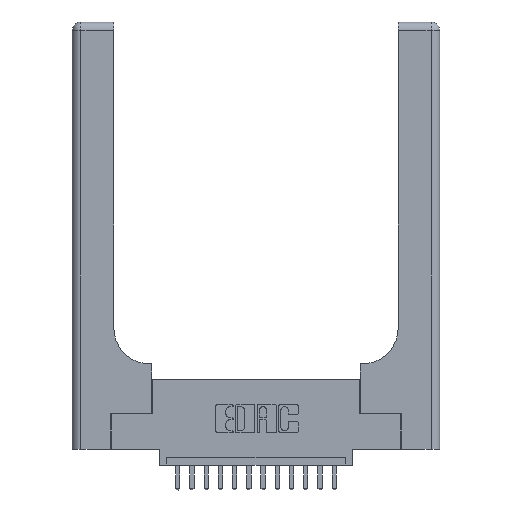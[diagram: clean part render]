
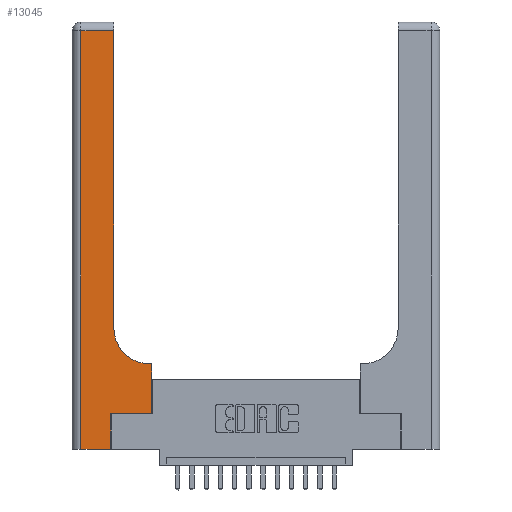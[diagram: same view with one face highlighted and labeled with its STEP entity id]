
A CAD part, top view. The second image highlights one B-rep face of the part: STEP entity #13045.
In plain terms, the highlighted planar face has unit normal (0, 0, 1).
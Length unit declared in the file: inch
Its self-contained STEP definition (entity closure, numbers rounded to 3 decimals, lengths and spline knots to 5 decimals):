
#655 = VERTEX_POINT ( 'NONE', #3529 ) ;
#848 = CARTESIAN_POINT ( 'NONE',  ( 0., 0., 0.37 ) ) ;
#951 = CARTESIAN_POINT ( 'NONE',  ( 0.269, 0.25, 0.37 ) ) ;
#1028 = ORIENTED_EDGE ( 'NONE', *, *, #3566, .T. ) ;
#1080 = CIRCLE ( 'NONE', #16007, 0.25 ) ;
#1304 = FACE_OUTER_BOUND ( 'NONE', #6189, .T. ) ;
#1462 = VERTEX_POINT ( 'NONE', #9787 ) ;
#1729 = VERTEX_POINT ( 'NONE', #15206 ) ;
#1758 = ORIENTED_EDGE ( 'NONE', *, *, #6445, .T. ) ;
#1901 = CARTESIAN_POINT ( 'NONE',  ( 0.2915, 0.85, 0.37 ) ) ;
#1990 = DIRECTION ( 'NONE',  ( 1., 0., 0. ) ) ;
#3059 = DIRECTION ( 'NONE',  ( 0., -1., 0. ) ) ;
#3529 = CARTESIAN_POINT ( 'NONE',  ( 0.5585, 0.6, 0.37 ) ) ;
#3566 = EDGE_CURVE ( 'NONE', #11790, #1729, #3611, .T. ) ;
#3611 = LINE ( 'NONE', #18075, #12315 ) ;
#4574 = DIRECTION ( 'NONE',  ( 0., 1., 0. ) ) ;
#4663 = VECTOR ( 'NONE', #6297, 39.37008 ) ;
#4793 = CARTESIAN_POINT ( 'NONE',  ( 0.2915, 0.6, 0.37 ) ) ;
#5058 = CARTESIAN_POINT ( 'NONE',  ( 0.269, 0., 0.37 ) ) ;
#5622 = ORIENTED_EDGE ( 'NONE', *, *, #17671, .T. ) ;
#6080 = VECTOR ( 'NONE', #11814, 39.37008 ) ;
#6189 = EDGE_LOOP ( 'NONE', ( #5622, #1758, #10325, #6398, #13712, #1028, #14439, #16842, #10997 ) ) ;
#6202 = LINE ( 'NONE', #12095, #4663 ) ;
#6297 = DIRECTION ( 'NONE',  ( -1., 0., 0. ) ) ;
#6398 = ORIENTED_EDGE ( 'NONE', *, *, #15666, .T. ) ;
#6416 = AXIS2_PLACEMENT_3D ( 'NONE', #9913, #12933, #11415 ) ;
#6445 = EDGE_CURVE ( 'NONE', #7885, #12751, #6202, .T. ) ;
#7050 = VECTOR ( 'NONE', #17914, 39.37008 ) ;
#7479 = VECTOR ( 'NONE', #3059, 39.37008 ) ;
#7856 = CARTESIAN_POINT ( 'NONE',  ( 0.5585, 0.25, 0.37 ) ) ;
#7885 = VERTEX_POINT ( 'NONE', #10711 ) ;
#7977 = DIRECTION ( 'NONE',  ( 0., 1., 0. ) ) ;
#8329 = EDGE_CURVE ( 'NONE', #12751, #1462, #11925, .T. ) ;
#8510 = PLANE ( 'NONE',  #6416 ) ;
#8682 = CARTESIAN_POINT ( 'NONE',  ( 0.2915, 3., 0.37 ) ) ;
#9111 = DIRECTION ( 'NONE',  ( 0., 0., -1. ) ) ;
#9163 = CARTESIAN_POINT ( 'NONE',  ( 0.5415, 0.85, 0.37 ) ) ;
#9478 = EDGE_CURVE ( 'NONE', #15813, #11790, #11890, .T. ) ;
#9787 = CARTESIAN_POINT ( 'NONE',  ( 0.06, 0., 0.37 ) ) ;
#9854 = LINE ( 'NONE', #4793, #6080 ) ;
#9913 = CARTESIAN_POINT ( 'NONE',  ( 0., 3., 0.37 ) ) ;
#9914 = CARTESIAN_POINT ( 'NONE',  ( 0.269, 0., 0.37 ) ) ;
#10059 = DIRECTION ( 'NONE',  ( 1., 0., 0. ) ) ;
#10113 = CARTESIAN_POINT ( 'NONE',  ( 0.06, 3., 0.37 ) ) ;
#10325 = ORIENTED_EDGE ( 'NONE', *, *, #8329, .T. ) ;
#10711 = CARTESIAN_POINT ( 'NONE',  ( 0.2915, 2.94, 0.37 ) ) ;
#10997 = ORIENTED_EDGE ( 'NONE', *, *, #13299, .T. ) ;
#11036 = DIRECTION ( 'NONE',  ( 1., 0., 0. ) ) ;
#11415 = DIRECTION ( 'NONE',  ( -1., 0., 0. ) ) ;
#11704 = VERTEX_POINT ( 'NONE', #11883 ) ;
#11790 = VERTEX_POINT ( 'NONE', #951 ) ;
#11814 = DIRECTION ( 'NONE',  ( -1., 0., 0. ) ) ;
#11883 = CARTESIAN_POINT ( 'NONE',  ( 0.5415, 0.6, 0.37 ) ) ;
#11890 = LINE ( 'NONE', #5058, #13260 ) ;
#11925 = LINE ( 'NONE', #10113, #7479 ) ;
#12095 = CARTESIAN_POINT ( 'NONE',  ( 0., 2.94, 0.37 ) ) ;
#12315 = VECTOR ( 'NONE', #10059, 39.37008 ) ;
#12751 = VERTEX_POINT ( 'NONE', #14860 ) ;
#12933 = DIRECTION ( 'NONE',  ( 0., 0., -1. ) ) ;
#13045 = ADVANCED_FACE ( 'NONE', ( #1304 ), #8510, .F. ) ;
#13260 = VECTOR ( 'NONE', #7977, 39.37008 ) ;
#13299 = EDGE_CURVE ( 'NONE', #11704, #18476, #1080, .T. ) ;
#13712 = ORIENTED_EDGE ( 'NONE', *, *, #9478, .T. ) ;
#14166 = EDGE_CURVE ( 'NONE', #655, #11704, #9854, .T. ) ;
#14439 = ORIENTED_EDGE ( 'NONE', *, *, #16186, .T. ) ;
#14648 = LINE ( 'NONE', #7856, #7050 ) ;
#14860 = CARTESIAN_POINT ( 'NONE',  ( 0.06, 2.94, 0.37 ) ) ;
#15021 = LINE ( 'NONE', #8682, #16586 ) ;
#15206 = CARTESIAN_POINT ( 'NONE',  ( 0.5585, 0.25, 0.37 ) ) ;
#15666 = EDGE_CURVE ( 'NONE', #1462, #15813, #16229, .T. ) ;
#15813 = VERTEX_POINT ( 'NONE', #9914 ) ;
#16007 = AXIS2_PLACEMENT_3D ( 'NONE', #9163, #9111, #1990 ) ;
#16186 = EDGE_CURVE ( 'NONE', #1729, #655, #14648, .T. ) ;
#16229 = LINE ( 'NONE', #848, #17347 ) ;
#16586 = VECTOR ( 'NONE', #4574, 39.37008 ) ;
#16842 = ORIENTED_EDGE ( 'NONE', *, *, #14166, .T. ) ;
#17347 = VECTOR ( 'NONE', #11036, 39.37008 ) ;
#17671 = EDGE_CURVE ( 'NONE', #18476, #7885, #15021, .T. ) ;
#17914 = DIRECTION ( 'NONE',  ( 0., 1., 0. ) ) ;
#18075 = CARTESIAN_POINT ( 'NONE',  ( 0.269, 0.25, 0.37 ) ) ;
#18476 = VERTEX_POINT ( 'NONE', #1901 ) ;
